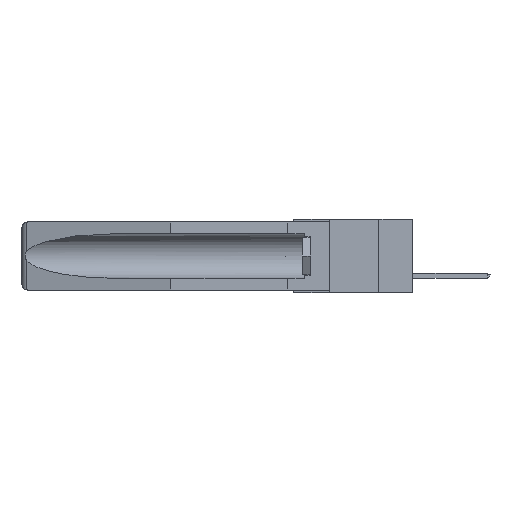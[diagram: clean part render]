
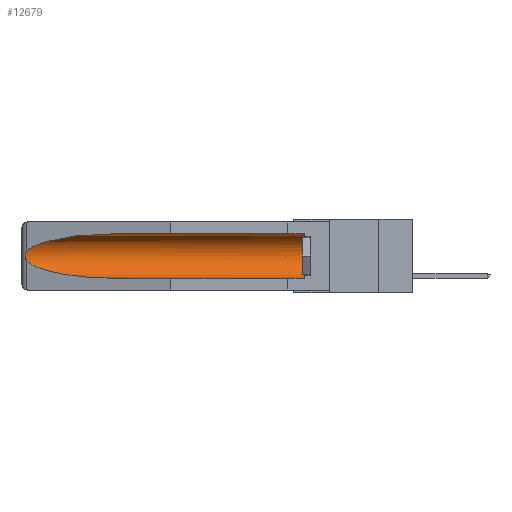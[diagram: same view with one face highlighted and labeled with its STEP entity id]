
A CAD part, left-side view. The second image highlights one B-rep face of the part: STEP entity #12679.
In plain terms, the highlighted cylindrical face has radius 2.857 mm (diameter 5.715 mm), a partial arc.
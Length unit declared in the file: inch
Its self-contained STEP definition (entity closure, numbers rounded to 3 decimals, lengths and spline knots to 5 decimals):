
#366 = CARTESIAN_POINT ( 'NONE',  ( 0.155, 1.07973, -0.284 ) ) ;
#496 = CARTESIAN_POINT ( 'NONE',  ( 0.155, 1.07973, -0.059 ) ) ;
#565 = DIRECTION ( 'NONE',  ( 0., 1., 0. ) ) ;
#871 = AXIS2_PLACEMENT_3D ( 'NONE', #10886, #5970, #24128 ) ;
#975 = CARTESIAN_POINT ( 'NONE',  ( 0.26655, 1.53094, -0.18657 ) ) ;
#1321 = CARTESIAN_POINT ( 'NONE',  ( 0.26537, 1.52718, -0.19328 ) ) ;
#2313 = ORIENTED_EDGE ( 'NONE', *, *, #30804, .F. ) ;
#2795 = CIRCLE ( 'NONE', #9894, 0.1125 ) ;
#3606 = CARTESIAN_POINT ( 'NONE',  ( 0.26654, 1.53092, -0.15636 ) ) ;
#4657 =( BOUNDED_CURVE ( )  B_SPLINE_CURVE ( 3, ( #29009, #8281, #16033, #366 ),
 .UNSPECIFIED., .F., .F. ) 
 B_SPLINE_CURVE_WITH_KNOTS ( ( 4, 4 ),
 ( 0.1948, 1.5708 ),
 .UNSPECIFIED. ) 
 CURVE ( )  GEOMETRIC_REPRESENTATION_ITEM ( )  RATIONAL_B_SPLINE_CURVE ( ( 1., 0.848, 0.848, 1. ) ) 
 REPRESENTATION_ITEM ( '' )  );
#4870 = VERTEX_POINT ( 'NONE', #33301 ) ;
#5970 = DIRECTION ( 'NONE',  ( 0., 1., 0. ) ) ;
#5983 = VECTOR ( 'NONE', #8326, 39.37008 ) ;
#6699 = VERTEX_POINT ( 'NONE', #496 ) ;
#6832 = ORIENTED_EDGE ( 'NONE', *, *, #24510, .T. ) ;
#7786 = CYLINDRICAL_SURFACE ( 'NONE', #871, 0.1125 ) ;
#8006 = VECTOR ( 'NONE', #565, 39.37008 ) ;
#8281 = CARTESIAN_POINT ( 'NONE',  ( 0.25451, 1.48313, -0.24835 ) ) ;
#8326 = DIRECTION ( 'NONE',  ( 0., 1., 0. ) ) ;
#8550 = VERTEX_POINT ( 'NONE', #29230 ) ;
#9858 = EDGE_CURVE ( 'NONE', #4870, #6699, #14930, .T. ) ;
#9894 = AXIS2_PLACEMENT_3D ( 'NONE', #30583, #14968, #17260 ) ;
#10096 = CARTESIAN_POINT ( 'NONE',  ( 0.155, 1.07973, -0.284 ) ) ;
#10444 = CARTESIAN_POINT ( 'NONE',  ( 0.26537, 1.52718, -0.14972 ) ) ;
#10886 = CARTESIAN_POINT ( 'NONE',  ( 0.155, -0.30754, -0.1715 ) ) ;
#11094 = CARTESIAN_POINT ( 'NONE',  ( 0.155, -0.30754, -0.059 ) ) ;
#12628 = CARTESIAN_POINT ( 'NONE',  ( 0.21114, 1.30732, -0.059 ) ) ;
#12679 = ADVANCED_FACE ( 'NONE', ( #16747 ), #7786, .F. ) ;
#13915 = CARTESIAN_POINT ( 'NONE',  ( 0.2675, 1.53308, -0.17534 ) ) ;
#13917 = EDGE_CURVE ( 'NONE', #14646, #4870, #2795, .T. ) ;
#14029 = CARTESIAN_POINT ( 'NONE',  ( 0.26597, 1.52961, -0.15275 ) ) ;
#14646 = VERTEX_POINT ( 'NONE', #20449 ) ;
#14719 = VERTEX_POINT ( 'NONE', #10096 ) ;
#14930 = LINE ( 'NONE', #11094, #8006 ) ;
#14968 = DIRECTION ( 'NONE',  ( 0., -1., 0. ) ) ;
#16033 = CARTESIAN_POINT ( 'NONE',  ( 0.21114, 1.30732, -0.284 ) ) ;
#16654 = CARTESIAN_POINT ( 'NONE',  ( 0.26597, 1.5296, -0.19026 ) ) ;
#16747 = FACE_OUTER_BOUND ( 'NONE', #28501, .T. ) ;
#16849 = CARTESIAN_POINT ( 'NONE',  ( 0.26537, 1.52718, -0.19328 ) ) ;
#16877 = CARTESIAN_POINT ( 'NONE',  ( 0.2673, 1.53269, -0.17917 ) ) ;
#17238 =( BOUNDED_CURVE ( )  B_SPLINE_CURVE ( 3, ( #26889, #12628, #23462, #10444 ),
 .UNSPECIFIED., .F., .F. ) 
 B_SPLINE_CURVE_WITH_KNOTS ( ( 4, 4 ),
 ( 4.71239, 6.08839 ),
 .UNSPECIFIED. ) 
 CURVE ( )  GEOMETRIC_REPRESENTATION_ITEM ( )  RATIONAL_B_SPLINE_CURVE ( ( 1., 0.848, 0.848, 1. ) ) 
 REPRESENTATION_ITEM ( '' )  );
#17260 = DIRECTION ( 'NONE',  ( 0., 0., 1. ) ) ;
#18414 = EDGE_CURVE ( 'NONE', #22750, #14719, #4657, .T. ) ;
#19472 = CARTESIAN_POINT ( 'NONE',  ( 0.2673, 1.5327, -0.16383 ) ) ;
#19849 = LINE ( 'NONE', #31134, #5983 ) ;
#20449 = CARTESIAN_POINT ( 'NONE',  ( 0.155, 0.126, -0.284 ) ) ;
#21645 = CARTESIAN_POINT ( 'NONE',  ( 0.26537, 1.52718, -0.14972 ) ) ;
#21977 = CARTESIAN_POINT ( 'NONE',  ( 0.2675, 1.53308, -0.16763 ) ) ;
#22153 = ORIENTED_EDGE ( 'NONE', *, *, #9858, .T. ) ;
#22220 = B_SPLINE_CURVE_WITH_KNOTS ( 'NONE', 3,
 ( #21645, #14029, #3606, #19472, #21977, #13915, #16877, #975, #16654, #1321 ),
 .UNSPECIFIED., .F., .F.,
 ( 4, 2, 2, 2, 4 ),
 ( 0., 0.00029, 0.00058, 0.00087, 0.00117 ),
 .UNSPECIFIED. ) ;
#22750 = VERTEX_POINT ( 'NONE', #16849 ) ;
#23433 = ORIENTED_EDGE ( 'NONE', *, *, #13917, .T. ) ;
#23462 = CARTESIAN_POINT ( 'NONE',  ( 0.25451, 1.48313, -0.09465 ) ) ;
#23799 = ORIENTED_EDGE ( 'NONE', *, *, #31648, .T. ) ;
#24128 = DIRECTION ( 'NONE',  ( 0., 0., 1. ) ) ;
#24510 = EDGE_CURVE ( 'NONE', #8550, #22750, #22220, .T. ) ;
#26889 = CARTESIAN_POINT ( 'NONE',  ( 0.155, 1.07973, -0.059 ) ) ;
#27252 = ORIENTED_EDGE ( 'NONE', *, *, #18414, .T. ) ;
#28501 = EDGE_LOOP ( 'NONE', ( #23799, #6832, #27252, #2313, #23433, #22153 ) ) ;
#29009 = CARTESIAN_POINT ( 'NONE',  ( 0.26537, 1.52718, -0.19328 ) ) ;
#29230 = CARTESIAN_POINT ( 'NONE',  ( 0.26537, 1.52718, -0.14972 ) ) ;
#30583 = CARTESIAN_POINT ( 'NONE',  ( 0.155, 0.126, -0.1715 ) ) ;
#30804 = EDGE_CURVE ( 'NONE', #14646, #14719, #19849, .T. ) ;
#31134 = CARTESIAN_POINT ( 'NONE',  ( 0.155, -0.30754, -0.284 ) ) ;
#31648 = EDGE_CURVE ( 'NONE', #6699, #8550, #17238, .T. ) ;
#33301 = CARTESIAN_POINT ( 'NONE',  ( 0.155, 0.126, -0.059 ) ) ;
